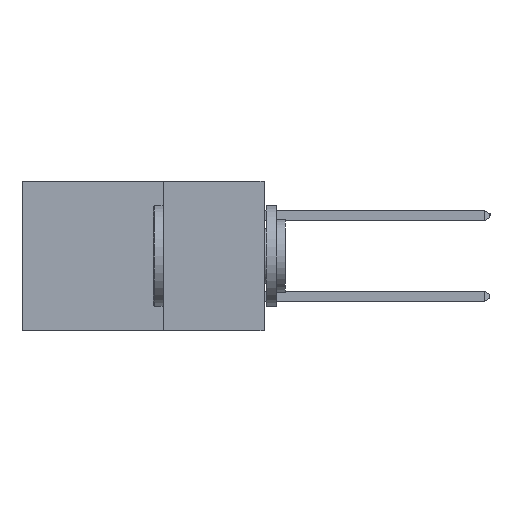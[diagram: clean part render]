
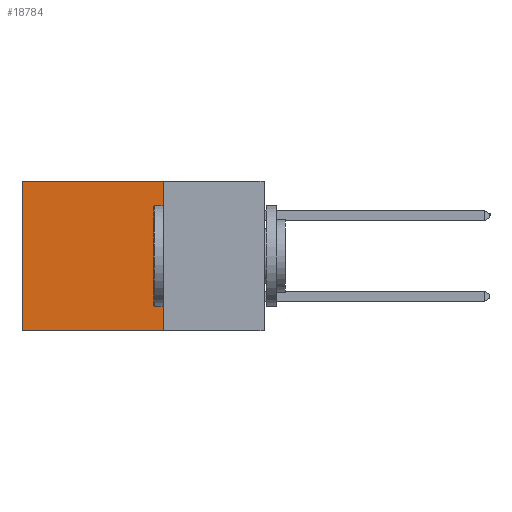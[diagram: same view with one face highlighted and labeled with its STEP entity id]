
A CAD part, left-side view. The second image highlights one B-rep face of the part: STEP entity #18784.
In plain terms, the highlighted planar face has unit normal (-1, 0, 0).
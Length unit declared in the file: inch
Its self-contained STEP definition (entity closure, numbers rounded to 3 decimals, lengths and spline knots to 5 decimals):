
#42 = EDGE_LOOP ( 'NONE', ( #16645, #6112, #7065, #13662 ) ) ;
#683 = EDGE_CURVE ( 'NONE', #15599, #4991, #1221, .T. ) ;
#718 = PLANE ( 'NONE',  #13350 ) ;
#1058 = CARTESIAN_POINT ( 'NONE',  ( 0.2615, 0.6, -0.37 ) ) ;
#1221 = LINE ( 'NONE', #19104, #16151 ) ;
#2125 = EDGE_CURVE ( 'NONE', #9331, #7990, #19414, .T. ) ;
#2209 = DIRECTION ( 'NONE',  ( 0., 0., -1. ) ) ;
#2601 = CARTESIAN_POINT ( 'NONE',  ( 0.2615, 0.25, -0.37 ) ) ;
#2888 = VECTOR ( 'NONE', #12591, 39.37008 ) ;
#3722 = VECTOR ( 'NONE', #19130, 39.37008 ) ;
#4103 = DIRECTION ( 'NONE',  ( 0., 1., 0. ) ) ;
#4964 = FACE_OUTER_BOUND ( 'NONE', #42, .T. ) ;
#4991 = VERTEX_POINT ( 'NONE', #1058 ) ;
#5649 = EDGE_CURVE ( 'NONE', #7990, #4991, #10355, .T. ) ;
#6112 = ORIENTED_EDGE ( 'NONE', *, *, #5649, .F. ) ;
#7065 = ORIENTED_EDGE ( 'NONE', *, *, #2125, .F. ) ;
#7990 = VERTEX_POINT ( 'NONE', #2601 ) ;
#9331 = VERTEX_POINT ( 'NONE', #12859 ) ;
#9633 = LINE ( 'NONE', #18668, #2888 ) ;
#9936 = EDGE_CURVE ( 'NONE', #9331, #15599, #9633, .T. ) ;
#10355 = LINE ( 'NONE', #10441, #12982 ) ;
#10441 = CARTESIAN_POINT ( 'NONE',  ( 0.2615, 0.25, -0.37 ) ) ;
#10833 = DIRECTION ( 'NONE',  ( 1., 0., 0. ) ) ;
#11827 = CARTESIAN_POINT ( 'NONE',  ( 0.2615, 0.6, 0. ) ) ;
#12465 = DIRECTION ( 'NONE',  ( 0., 0., -1. ) ) ;
#12591 = DIRECTION ( 'NONE',  ( 0., 1., 0. ) ) ;
#12859 = CARTESIAN_POINT ( 'NONE',  ( 0.2615, 0.25, 0. ) ) ;
#12982 = VECTOR ( 'NONE', #4103, 39.37008 ) ;
#13350 = AXIS2_PLACEMENT_3D ( 'NONE', #15711, #10833, #2209 ) ;
#13662 = ORIENTED_EDGE ( 'NONE', *, *, #9936, .T. ) ;
#15599 = VERTEX_POINT ( 'NONE', #11827 ) ;
#15711 = CARTESIAN_POINT ( 'NONE',  ( 0.2615, 0.25, -0.37 ) ) ;
#16151 = VECTOR ( 'NONE', #12465, 39.37008 ) ;
#16645 = ORIENTED_EDGE ( 'NONE', *, *, #683, .T. ) ;
#17639 = CARTESIAN_POINT ( 'NONE',  ( 0.2615, 0.25, -0.37 ) ) ;
#18668 = CARTESIAN_POINT ( 'NONE',  ( 0.2615, 0.25, 0. ) ) ;
#18784 = ADVANCED_FACE ( 'NONE', ( #4964 ), #718, .F. ) ;
#19104 = CARTESIAN_POINT ( 'NONE',  ( 0.2615, 0.6, -0.37 ) ) ;
#19130 = DIRECTION ( 'NONE',  ( 0., 0., -1. ) ) ;
#19414 = LINE ( 'NONE', #17639, #3722 ) ;
